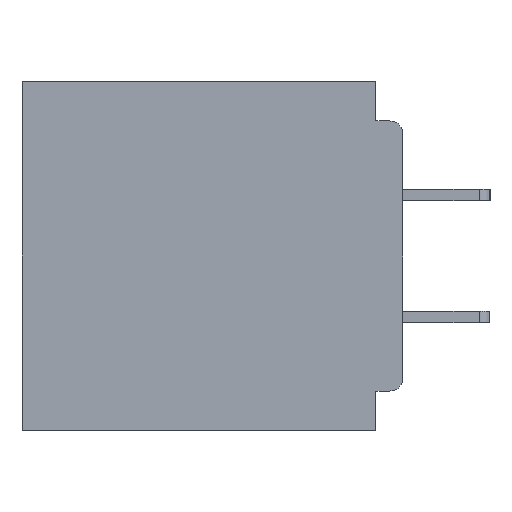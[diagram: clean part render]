
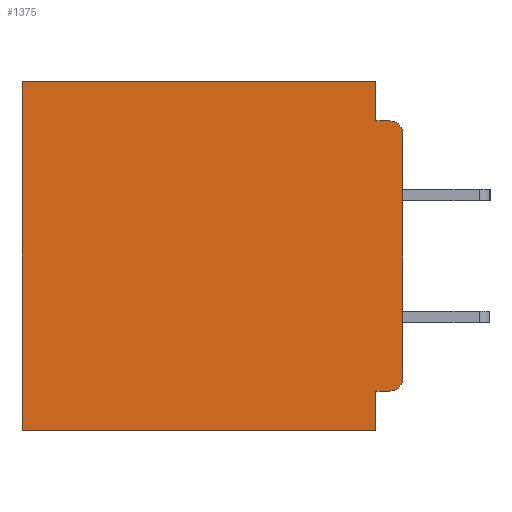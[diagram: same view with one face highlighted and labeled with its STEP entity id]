
A CAD part, left-side view. The second image highlights one B-rep face of the part: STEP entity #1375.
In plain terms, the highlighted planar face has unit normal (-1, 0, 0).
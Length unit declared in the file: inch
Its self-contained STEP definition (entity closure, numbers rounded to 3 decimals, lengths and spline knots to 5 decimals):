
#392 = CARTESIAN_POINT ( 'NONE',  ( 0.3, 0., -0.4 ) ) ;
#1375 = ADVANCED_FACE ( 'NONE', ( #24628 ), #5213, .F. ) ;
#1728 = DIRECTION ( 'NONE',  ( -1., 0., 0. ) ) ;
#2682 = VERTEX_POINT ( 'NONE', #25607 ) ;
#2781 = DIRECTION ( 'NONE',  ( 0., 0., -1. ) ) ;
#2988 = CARTESIAN_POINT ( 'NONE',  ( 0.3, 0.437, -0.4 ) ) ;
#3176 = CARTESIAN_POINT ( 'NONE',  ( 0.3, 0.437, 0. ) ) ;
#4348 = EDGE_CURVE ( 'NONE', #6641, #44225, #43729, .T. ) ;
#5213 = PLANE ( 'NONE',  #40824 ) ;
#5331 = CARTESIAN_POINT ( 'NONE',  ( 0.3, 0., -0.4 ) ) ;
#5471 = EDGE_CURVE ( 'NONE', #44225, #40788, #13718, .T. ) ;
#5971 = DIRECTION ( 'NONE',  ( 0., 0., -1. ) ) ;
#6641 = VERTEX_POINT ( 'NONE', #19448 ) ;
#7239 = CARTESIAN_POINT ( 'NONE',  ( 0.3, 0., -0.355 ) ) ;
#7943 = LINE ( 'NONE', #2988, #37254 ) ;
#8335 = CARTESIAN_POINT ( 'NONE',  ( 0.3, 0.015, -0.355 ) ) ;
#9041 = VERTEX_POINT ( 'NONE', #34313 ) ;
#9252 = ORIENTED_EDGE ( 'NONE', *, *, #39887, .F. ) ;
#9950 = CARTESIAN_POINT ( 'NONE',  ( 0.3, 0., -0.4 ) ) ;
#10291 = CARTESIAN_POINT ( 'NONE',  ( 0.3, 0.031, -0.4 ) ) ;
#10355 = VECTOR ( 'NONE', #11065, 39.37008 ) ;
#11065 = DIRECTION ( 'NONE',  ( 0., 1., 0. ) ) ;
#11406 = EDGE_CURVE ( 'NONE', #13550, #18167, #7943, .T. ) ;
#11825 = CIRCLE ( 'NONE', #14955, 0.015 ) ;
#12532 = VECTOR ( 'NONE', #39146, 39.37008 ) ;
#13441 = CARTESIAN_POINT ( 'NONE',  ( 0.3, 0., -0.06 ) ) ;
#13550 = VERTEX_POINT ( 'NONE', #3176 ) ;
#13718 = LINE ( 'NONE', #39530, #12532 ) ;
#14147 = CARTESIAN_POINT ( 'NONE',  ( 0.3, 0., 0. ) ) ;
#14729 = DIRECTION ( 'NONE',  ( -1., 0., 0. ) ) ;
#14955 = AXIS2_PLACEMENT_3D ( 'NONE', #37006, #1728, #28533 ) ;
#15759 = ORIENTED_EDGE ( 'NONE', *, *, #49483, .T. ) ;
#17296 = EDGE_CURVE ( 'NONE', #32441, #40788, #37901, .T. ) ;
#18167 = VERTEX_POINT ( 'NONE', #49223 ) ;
#18218 = ORIENTED_EDGE ( 'NONE', *, *, #17296, .T. ) ;
#19448 = CARTESIAN_POINT ( 'NONE',  ( 0.3, 0.031, 0. ) ) ;
#19587 = CARTESIAN_POINT ( 'NONE',  ( 0.3, 0.015, -0.045 ) ) ;
#21005 = ORIENTED_EDGE ( 'NONE', *, *, #5471, .F. ) ;
#21588 = ORIENTED_EDGE ( 'NONE', *, *, #46161, .F. ) ;
#22293 = VECTOR ( 'NONE', #23270, 39.37008 ) ;
#23270 = DIRECTION ( 'NONE',  ( 0., 0., -1. ) ) ;
#24081 = EDGE_CURVE ( 'NONE', #32441, #2682, #46097, .T. ) ;
#24628 = FACE_OUTER_BOUND ( 'NONE', #34799, .T. ) ;
#25563 = ORIENTED_EDGE ( 'NONE', *, *, #33767, .T. ) ;
#25607 = CARTESIAN_POINT ( 'NONE',  ( 0.3, 0., -0.34 ) ) ;
#26542 = CARTESIAN_POINT ( 'NONE',  ( 0.3, 0.031, 0. ) ) ;
#27038 = ORIENTED_EDGE ( 'NONE', *, *, #11406, .T. ) ;
#27541 = VECTOR ( 'NONE', #37066, 39.37008 ) ;
#28213 = VECTOR ( 'NONE', #2781, 39.37008 ) ;
#28533 = DIRECTION ( 'NONE',  ( 0., 0., -1. ) ) ;
#28758 = LINE ( 'NONE', #14147, #27541 ) ;
#32030 = VECTOR ( 'NONE', #43529, 39.37008 ) ;
#32441 = VERTEX_POINT ( 'NONE', #13441 ) ;
#33205 = LINE ( 'NONE', #5331, #32030 ) ;
#33497 = CARTESIAN_POINT ( 'NONE',  ( 0.3, 0.031, -0.045 ) ) ;
#33673 = ORIENTED_EDGE ( 'NONE', *, *, #24081, .F. ) ;
#33767 = EDGE_CURVE ( 'NONE', #6641, #13550, #28758, .T. ) ;
#34313 = CARTESIAN_POINT ( 'NONE',  ( 0.3, 0.031, -0.4 ) ) ;
#34799 = EDGE_LOOP ( 'NONE', ( #33673, #18218, #21005, #37221, #25563, #27038, #9252, #35675, #21588, #15759 ) ) ;
#35556 = VERTEX_POINT ( 'NONE', #36695 ) ;
#35675 = ORIENTED_EDGE ( 'NONE', *, *, #47383, .F. ) ;
#36011 = VECTOR ( 'NONE', #42464, 39.37008 ) ;
#36695 = CARTESIAN_POINT ( 'NONE',  ( 0.3, 0.031, -0.355 ) ) ;
#37006 = CARTESIAN_POINT ( 'NONE',  ( 0.3, 0.015, -0.34 ) ) ;
#37066 = DIRECTION ( 'NONE',  ( 0., 1., 0. ) ) ;
#37221 = ORIENTED_EDGE ( 'NONE', *, *, #4348, .F. ) ;
#37254 = VECTOR ( 'NONE', #48691, 39.37008 ) ;
#37653 = CARTESIAN_POINT ( 'NONE',  ( 0.3, 0.015, -0.06 ) ) ;
#37901 = CIRCLE ( 'NONE', #42078, 0.015 ) ;
#38304 = LINE ( 'NONE', #10291, #28213 ) ;
#39146 = DIRECTION ( 'NONE',  ( 0., -1., 0. ) ) ;
#39267 = DIRECTION ( 'NONE',  ( 1., 0., 0. ) ) ;
#39530 = CARTESIAN_POINT ( 'NONE',  ( 0.3, 0., -0.045 ) ) ;
#39887 = EDGE_CURVE ( 'NONE', #9041, #18167, #33205, .T. ) ;
#40788 = VERTEX_POINT ( 'NONE', #19587 ) ;
#40824 = AXIS2_PLACEMENT_3D ( 'NONE', #9950, #39267, #5971 ) ;
#40837 = LINE ( 'NONE', #7239, #10355 ) ;
#41456 = DIRECTION ( 'NONE',  ( 0., 0., -1. ) ) ;
#42078 = AXIS2_PLACEMENT_3D ( 'NONE', #37653, #14729, #41456 ) ;
#42464 = DIRECTION ( 'NONE',  ( 0., 0., -1. ) ) ;
#42682 = VERTEX_POINT ( 'NONE', #8335 ) ;
#43529 = DIRECTION ( 'NONE',  ( 0., 1., 0. ) ) ;
#43729 = LINE ( 'NONE', #26542, #22293 ) ;
#44225 = VERTEX_POINT ( 'NONE', #33497 ) ;
#46097 = LINE ( 'NONE', #392, #36011 ) ;
#46161 = EDGE_CURVE ( 'NONE', #42682, #35556, #40837, .T. ) ;
#47383 = EDGE_CURVE ( 'NONE', #35556, #9041, #38304, .T. ) ;
#48691 = DIRECTION ( 'NONE',  ( 0., 0., -1. ) ) ;
#49223 = CARTESIAN_POINT ( 'NONE',  ( 0.3, 0.437, -0.4 ) ) ;
#49483 = EDGE_CURVE ( 'NONE', #42682, #2682, #11825, .T. ) ;
